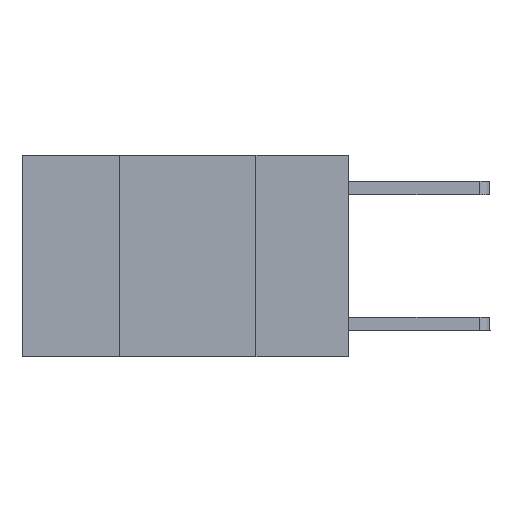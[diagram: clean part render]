
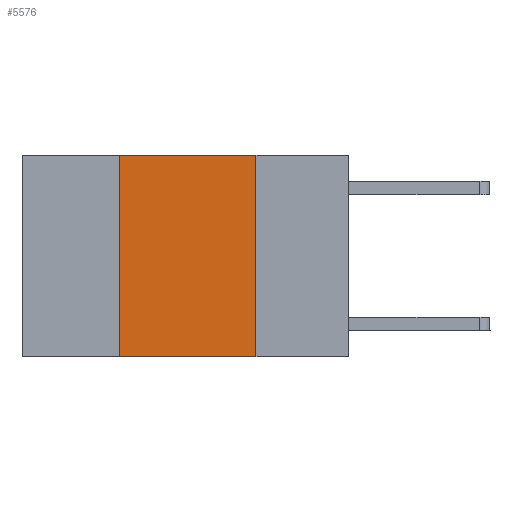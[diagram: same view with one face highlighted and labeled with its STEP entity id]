
A CAD part, left-side view. The second image highlights one B-rep face of the part: STEP entity #5576.
In plain terms, the highlighted planar face has unit normal (-1, 0, 0).
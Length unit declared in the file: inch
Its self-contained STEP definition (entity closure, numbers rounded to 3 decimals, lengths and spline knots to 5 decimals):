
#950 = CARTESIAN_POINT ( 'NONE',  ( 0., 0.42, 0. ) ) ;
#1570 = FACE_OUTER_BOUND ( 'NONE', #8087, .T. ) ;
#1937 = VERTEX_POINT ( 'NONE', #8027 ) ;
#2092 = EDGE_CURVE ( 'NONE', #3960, #4228, #6501, .T. ) ;
#2119 = CARTESIAN_POINT ( 'NONE',  ( 0., 0.6, -0.37 ) ) ;
#2230 = CARTESIAN_POINT ( 'NONE',  ( 0., 0.17, 0. ) ) ;
#2563 = CARTESIAN_POINT ( 'NONE',  ( 0., 0.17, 0. ) ) ;
#2968 = DIRECTION ( 'NONE',  ( 0., -1., 0. ) ) ;
#3066 = PLANE ( 'NONE',  #3316 ) ;
#3316 = AXIS2_PLACEMENT_3D ( 'NONE', #8640, #3856, #9371 ) ;
#3659 = VECTOR ( 'NONE', #7945, 39.37008 ) ;
#3856 = DIRECTION ( 'NONE',  ( 1., 0., 0. ) ) ;
#3960 = VERTEX_POINT ( 'NONE', #950 ) ;
#4228 = VERTEX_POINT ( 'NONE', #2563 ) ;
#5000 = ORIENTED_EDGE ( 'NONE', *, *, #7627, .T. ) ;
#5427 = LINE ( 'NONE', #2119, #7141 ) ;
#5494 = CARTESIAN_POINT ( 'NONE',  ( 0., 0.42, 0. ) ) ;
#5576 = ADVANCED_FACE ( 'NONE', ( #1570 ), #3066, .F. ) ;
#5797 = ORIENTED_EDGE ( 'NONE', *, *, #6235, .F. ) ;
#5833 = LINE ( 'NONE', #5494, #3659 ) ;
#6235 = EDGE_CURVE ( 'NONE', #4228, #9039, #6428, .T. ) ;
#6428 = LINE ( 'NONE', #2230, #7172 ) ;
#6501 = LINE ( 'NONE', #7284, #8286 ) ;
#6781 = ORIENTED_EDGE ( 'NONE', *, *, #7820, .F. ) ;
#7141 = VECTOR ( 'NONE', #2968, 39.37008 ) ;
#7172 = VECTOR ( 'NONE', #7912, 39.37008 ) ;
#7178 = ORIENTED_EDGE ( 'NONE', *, *, #2092, .F. ) ;
#7284 = CARTESIAN_POINT ( 'NONE',  ( 0., 0.6, 0. ) ) ;
#7627 = EDGE_CURVE ( 'NONE', #1937, #9039, #5427, .T. ) ;
#7820 = EDGE_CURVE ( 'NONE', #1937, #3960, #5833, .T. ) ;
#7912 = DIRECTION ( 'NONE',  ( 0., 0., -1. ) ) ;
#7945 = DIRECTION ( 'NONE',  ( 0., 0., 1. ) ) ;
#7959 = CARTESIAN_POINT ( 'NONE',  ( 0., 0.17, -0.37 ) ) ;
#8027 = CARTESIAN_POINT ( 'NONE',  ( 0., 0.42, -0.37 ) ) ;
#8087 = EDGE_LOOP ( 'NONE', ( #5797, #7178, #6781, #5000 ) ) ;
#8286 = VECTOR ( 'NONE', #9326, 39.37008 ) ;
#8640 = CARTESIAN_POINT ( 'NONE',  ( 0., 0.6, 0. ) ) ;
#9039 = VERTEX_POINT ( 'NONE', #7959 ) ;
#9326 = DIRECTION ( 'NONE',  ( 0., -1., 0. ) ) ;
#9371 = DIRECTION ( 'NONE',  ( 0., 0., -1. ) ) ;
